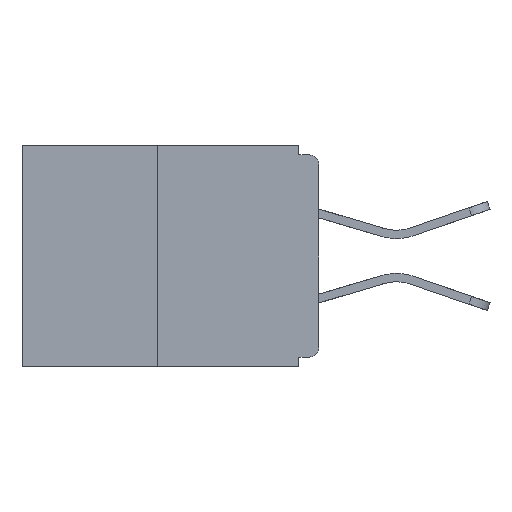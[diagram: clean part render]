
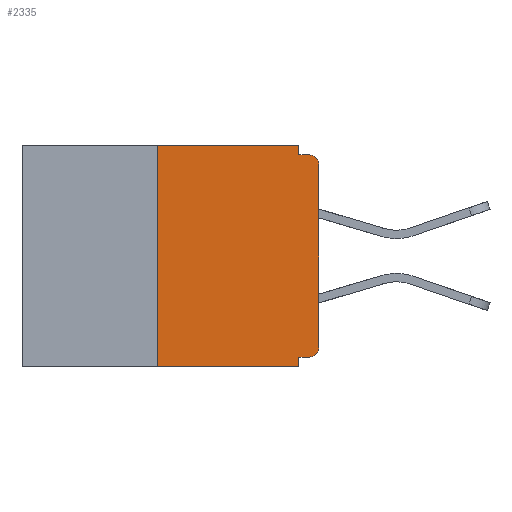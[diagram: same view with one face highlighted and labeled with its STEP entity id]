
A CAD part, left-side view. The second image highlights one B-rep face of the part: STEP entity #2335.
In plain terms, the highlighted planar face has unit normal (-1, 0, 0).
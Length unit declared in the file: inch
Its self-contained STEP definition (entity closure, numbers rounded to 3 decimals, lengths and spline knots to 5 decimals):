
#24 = CARTESIAN_POINT ( 'NONE',  ( 0., 0.015, -0.313 ) ) ;
#518 = CARTESIAN_POINT ( 'NONE',  ( 0., 0.015, -0.03 ) ) ;
#785 = AXIS2_PLACEMENT_3D ( 'NONE', #518, #3679, #5286 ) ;
#1394 = PLANE ( 'NONE',  #7879 ) ;
#1483 = CARTESIAN_POINT ( 'NONE',  ( 0., 0.46, 0. ) ) ;
#1553 = VERTEX_POINT ( 'NONE', #16956 ) ;
#1642 = DIRECTION ( 'NONE',  ( 0., 0., -1. ) ) ;
#1828 = LINE ( 'NONE', #16691, #15026 ) ;
#2335 = ADVANCED_FACE ( 'NONE', ( #11435 ), #1394, .F. ) ;
#2366 = CARTESIAN_POINT ( 'NONE',  ( 0., 0.25, -0.343 ) ) ;
#2734 = VECTOR ( 'NONE', #10482, 39.37008 ) ;
#2885 = CARTESIAN_POINT ( 'NONE',  ( 0., 0.25, 0. ) ) ;
#3009 = VERTEX_POINT ( 'NONE', #18158 ) ;
#3079 = DIRECTION ( 'NONE',  ( 1., 0., 0. ) ) ;
#3110 = DIRECTION ( 'NONE',  ( -1., 0., 0. ) ) ;
#3679 = DIRECTION ( 'NONE',  ( -1., 0., 0. ) ) ;
#3915 = LINE ( 'NONE', #20566, #6342 ) ;
#4200 = LINE ( 'NONE', #8125, #20570 ) ;
#4367 = EDGE_CURVE ( 'NONE', #1553, #3009, #17137, .T. ) ;
#4540 = LINE ( 'NONE', #1483, #19231 ) ;
#4554 = LINE ( 'NONE', #2885, #15288 ) ;
#4820 = DIRECTION ( 'NONE',  ( 0., -1., 0. ) ) ;
#5018 = VECTOR ( 'NONE', #18187, 39.37008 ) ;
#5033 = VERTEX_POINT ( 'NONE', #6452 ) ;
#5055 = LINE ( 'NONE', #15925, #15310 ) ;
#5286 = DIRECTION ( 'NONE',  ( 0., 0., -1. ) ) ;
#5338 = ORIENTED_EDGE ( 'NONE', *, *, #10138, .F. ) ;
#5843 = VERTEX_POINT ( 'NONE', #10051 ) ;
#6199 = ORIENTED_EDGE ( 'NONE', *, *, #7814, .T. ) ;
#6213 = DIRECTION ( 'NONE',  ( 0., 0., -1. ) ) ;
#6265 = ORIENTED_EDGE ( 'NONE', *, *, #13841, .F. ) ;
#6342 = VECTOR ( 'NONE', #11072, 39.37008 ) ;
#6368 = DIRECTION ( 'NONE',  ( 0., -1., 0. ) ) ;
#6402 = EDGE_LOOP ( 'NONE', ( #5338, #16879, #11820, #12955, #6265, #6199, #12759, #12446, #7033, #15699 ) ) ;
#6452 = CARTESIAN_POINT ( 'NONE',  ( 0., 0.031, 0. ) ) ;
#6846 = EDGE_CURVE ( 'NONE', #12719, #3009, #5055, .T. ) ;
#7033 = ORIENTED_EDGE ( 'NONE', *, *, #6846, .F. ) ;
#7235 = LINE ( 'NONE', #13405, #5018 ) ;
#7669 = VERTEX_POINT ( 'NONE', #2366 ) ;
#7814 = EDGE_CURVE ( 'NONE', #5843, #19759, #12087, .T. ) ;
#7879 = AXIS2_PLACEMENT_3D ( 'NONE', #15818, #3079, #6213 ) ;
#8125 = CARTESIAN_POINT ( 'NONE',  ( 0., 0., 0. ) ) ;
#8235 = CARTESIAN_POINT ( 'NONE',  ( 0., 0., -0.313 ) ) ;
#9749 = DIRECTION ( 'NONE',  ( 0., 0., 1. ) ) ;
#10051 = CARTESIAN_POINT ( 'NONE',  ( 0., 0.015, -0.328 ) ) ;
#10138 = EDGE_CURVE ( 'NONE', #12202, #5033, #4540, .T. ) ;
#10482 = DIRECTION ( 'NONE',  ( 0., 1., 0. ) ) ;
#11072 = DIRECTION ( 'NONE',  ( 0., -1., 0. ) ) ;
#11435 = FACE_OUTER_BOUND ( 'NONE', #6402, .T. ) ;
#11591 = EDGE_CURVE ( 'NONE', #7669, #12202, #4554, .T. ) ;
#11820 = ORIENTED_EDGE ( 'NONE', *, *, #15058, .T. ) ;
#11977 = EDGE_CURVE ( 'NONE', #17086, #15034, #1828, .T. ) ;
#12043 = EDGE_CURVE ( 'NONE', #5033, #12719, #7235, .T. ) ;
#12087 = CIRCLE ( 'NONE', #13915, 0.015 ) ;
#12202 = VERTEX_POINT ( 'NONE', #20112 ) ;
#12390 = DIRECTION ( 'NONE',  ( 0., 0., 1. ) ) ;
#12446 = ORIENTED_EDGE ( 'NONE', *, *, #4367, .T. ) ;
#12719 = VERTEX_POINT ( 'NONE', #17782 ) ;
#12759 = ORIENTED_EDGE ( 'NONE', *, *, #14202, .T. ) ;
#12955 = ORIENTED_EDGE ( 'NONE', *, *, #11977, .F. ) ;
#13405 = CARTESIAN_POINT ( 'NONE',  ( 0., 0.031, 0. ) ) ;
#13422 = CARTESIAN_POINT ( 'NONE',  ( 0., 0.031, -0.343 ) ) ;
#13552 = DIRECTION ( 'NONE',  ( 0., 0., -1. ) ) ;
#13841 = EDGE_CURVE ( 'NONE', #5843, #17086, #17163, .T. ) ;
#13915 = AXIS2_PLACEMENT_3D ( 'NONE', #24, #3110, #1642 ) ;
#14202 = EDGE_CURVE ( 'NONE', #19759, #1553, #4200, .T. ) ;
#15026 = VECTOR ( 'NONE', #13552, 39.37008 ) ;
#15034 = VERTEX_POINT ( 'NONE', #13422 ) ;
#15058 = EDGE_CURVE ( 'NONE', #7669, #15034, #3915, .T. ) ;
#15288 = VECTOR ( 'NONE', #12390, 39.37008 ) ;
#15310 = VECTOR ( 'NONE', #4820, 39.37008 ) ;
#15699 = ORIENTED_EDGE ( 'NONE', *, *, #12043, .F. ) ;
#15818 = CARTESIAN_POINT ( 'NONE',  ( 0., 0.46, 0. ) ) ;
#15925 = CARTESIAN_POINT ( 'NONE',  ( 0., 0., -0.015 ) ) ;
#16633 = CARTESIAN_POINT ( 'NONE',  ( 0., 0.031, -0.328 ) ) ;
#16691 = CARTESIAN_POINT ( 'NONE',  ( 0., 0.031, -0.343 ) ) ;
#16879 = ORIENTED_EDGE ( 'NONE', *, *, #11591, .F. ) ;
#16956 = CARTESIAN_POINT ( 'NONE',  ( 0., 0., -0.03 ) ) ;
#17086 = VERTEX_POINT ( 'NONE', #16633 ) ;
#17137 = CIRCLE ( 'NONE', #785, 0.015 ) ;
#17163 = LINE ( 'NONE', #20020, #2734 ) ;
#17782 = CARTESIAN_POINT ( 'NONE',  ( 0., 0.031, -0.015 ) ) ;
#18158 = CARTESIAN_POINT ( 'NONE',  ( 0., 0.015, -0.015 ) ) ;
#18187 = DIRECTION ( 'NONE',  ( 0., 0., -1. ) ) ;
#19231 = VECTOR ( 'NONE', #6368, 39.37008 ) ;
#19759 = VERTEX_POINT ( 'NONE', #8235 ) ;
#20020 = CARTESIAN_POINT ( 'NONE',  ( 0., 0., -0.328 ) ) ;
#20112 = CARTESIAN_POINT ( 'NONE',  ( 0., 0.25, 0. ) ) ;
#20566 = CARTESIAN_POINT ( 'NONE',  ( 0., 0.46, -0.343 ) ) ;
#20570 = VECTOR ( 'NONE', #9749, 39.37008 ) ;
